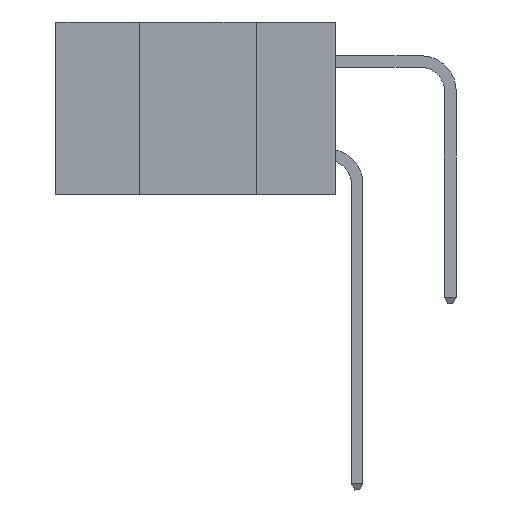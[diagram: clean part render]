
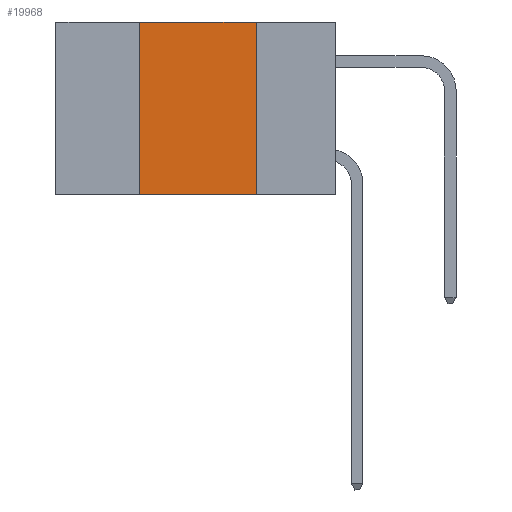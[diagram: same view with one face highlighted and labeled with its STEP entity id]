
A CAD part, left-side view. The second image highlights one B-rep face of the part: STEP entity #19968.
In plain terms, the highlighted planar face has unit normal (-1, 0, 0).
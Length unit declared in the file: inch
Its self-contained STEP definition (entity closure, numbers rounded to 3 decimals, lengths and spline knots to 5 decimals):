
#35 = ORIENTED_EDGE ( 'NONE', *, *, #22077, .T. ) ;
#530 = CARTESIAN_POINT ( 'NONE',  ( 0., 0.6, -0.37 ) ) ;
#881 = PLANE ( 'NONE',  #13019 ) ;
#908 = EDGE_LOOP ( 'NONE', ( #3126, #1647, #17513, #35 ) ) ;
#1615 = LINE ( 'NONE', #14979, #15058 ) ;
#1647 = ORIENTED_EDGE ( 'NONE', *, *, #7023, .F. ) ;
#2501 = EDGE_CURVE ( 'NONE', #6097, #9876, #1615, .T. ) ;
#2777 = CARTESIAN_POINT ( 'NONE',  ( 0., 0.17, -0.37 ) ) ;
#3126 = ORIENTED_EDGE ( 'NONE', *, *, #3305, .F. ) ;
#3305 = EDGE_CURVE ( 'NONE', #6468, #19271, #8619, .T. ) ;
#3463 = VECTOR ( 'NONE', #16297, 39.37008 ) ;
#4609 = DIRECTION ( 'NONE',  ( 1., 0., 0. ) ) ;
#4738 = VECTOR ( 'NONE', #11634, 39.37008 ) ;
#5071 = CARTESIAN_POINT ( 'NONE',  ( 0., 0.42, -0.37 ) ) ;
#5104 = CARTESIAN_POINT ( 'NONE',  ( 0., 0.17, 0. ) ) ;
#5306 = LINE ( 'NONE', #16590, #4738 ) ;
#6097 = VERTEX_POINT ( 'NONE', #5071 ) ;
#6468 = VERTEX_POINT ( 'NONE', #5104 ) ;
#6502 = DIRECTION ( 'NONE',  ( 0., 0., 1. ) ) ;
#7023 = EDGE_CURVE ( 'NONE', #9876, #6468, #5306, .T. ) ;
#8333 = LINE ( 'NONE', #530, #3463 ) ;
#8619 = LINE ( 'NONE', #20125, #16950 ) ;
#8937 = FACE_OUTER_BOUND ( 'NONE', #908, .T. ) ;
#9208 = CARTESIAN_POINT ( 'NONE',  ( 0., 0.42, 0. ) ) ;
#9876 = VERTEX_POINT ( 'NONE', #9208 ) ;
#11634 = DIRECTION ( 'NONE',  ( 0., -1., 0. ) ) ;
#13019 = AXIS2_PLACEMENT_3D ( 'NONE', #13278, #4609, #16606 ) ;
#13278 = CARTESIAN_POINT ( 'NONE',  ( 0., 0.6, 0. ) ) ;
#14979 = CARTESIAN_POINT ( 'NONE',  ( 0., 0.42, 0. ) ) ;
#15058 = VECTOR ( 'NONE', #6502, 39.37008 ) ;
#16297 = DIRECTION ( 'NONE',  ( 0., -1., 0. ) ) ;
#16590 = CARTESIAN_POINT ( 'NONE',  ( 0., 0.6, 0. ) ) ;
#16606 = DIRECTION ( 'NONE',  ( 0., 0., -1. ) ) ;
#16950 = VECTOR ( 'NONE', #21774, 39.37008 ) ;
#17513 = ORIENTED_EDGE ( 'NONE', *, *, #2501, .F. ) ;
#19271 = VERTEX_POINT ( 'NONE', #2777 ) ;
#19968 = ADVANCED_FACE ( 'NONE', ( #8937 ), #881, .F. ) ;
#20125 = CARTESIAN_POINT ( 'NONE',  ( 0., 0.17, 0. ) ) ;
#21774 = DIRECTION ( 'NONE',  ( 0., 0., -1. ) ) ;
#22077 = EDGE_CURVE ( 'NONE', #6097, #19271, #8333, .T. ) ;
